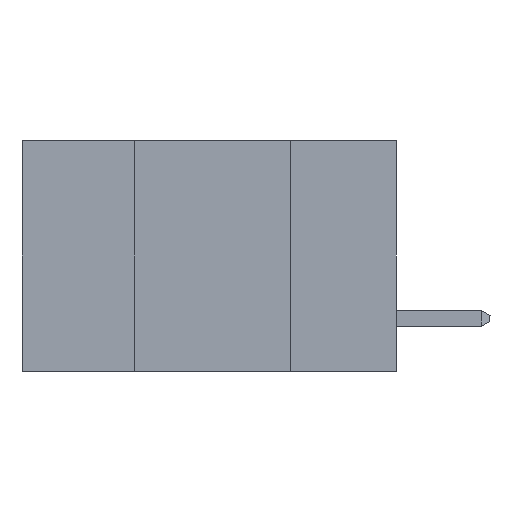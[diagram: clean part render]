
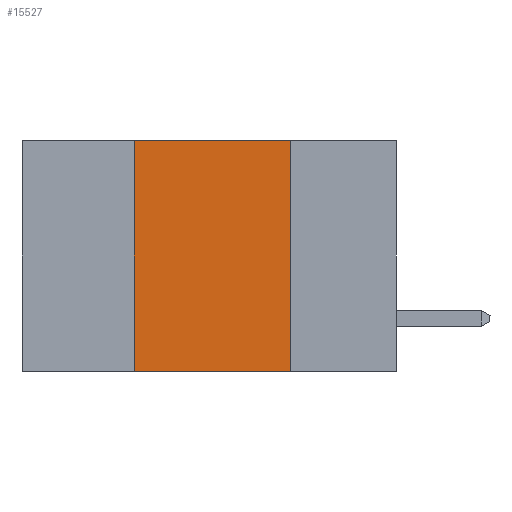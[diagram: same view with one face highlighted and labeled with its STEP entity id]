
A CAD part, left-side view. The second image highlights one B-rep face of the part: STEP entity #15527.
In plain terms, the highlighted planar face has unit normal (-1, 0, 0).
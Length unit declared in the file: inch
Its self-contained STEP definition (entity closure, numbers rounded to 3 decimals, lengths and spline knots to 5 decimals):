
#452 = VERTEX_POINT ( 'NONE', #5935 ) ;
#895 = DIRECTION ( 'NONE',  ( 0., 0., -1. ) ) ;
#1209 = DIRECTION ( 'NONE',  ( 0., 0., 1. ) ) ;
#1271 = CARTESIAN_POINT ( 'NONE',  ( 0., 0.42, -0.37 ) ) ;
#1286 = CARTESIAN_POINT ( 'NONE',  ( 0., 0.17, -0.37 ) ) ;
#2595 = AXIS2_PLACEMENT_3D ( 'NONE', #13153, #9141, #895 ) ;
#3821 = LINE ( 'NONE', #1271, #7104 ) ;
#4540 = ORIENTED_EDGE ( 'NONE', *, *, #9787, .F. ) ;
#4934 = FACE_OUTER_BOUND ( 'NONE', #7596, .T. ) ;
#5168 = VERTEX_POINT ( 'NONE', #16730 ) ;
#5935 = CARTESIAN_POINT ( 'NONE',  ( 0., 0.17, 0. ) ) ;
#6124 = VERTEX_POINT ( 'NONE', #9010 ) ;
#6601 = CARTESIAN_POINT ( 'NONE',  ( 0., 0.6, 0. ) ) ;
#6754 = CARTESIAN_POINT ( 'NONE',  ( 0., 0.6, -0.37 ) ) ;
#7034 = EDGE_CURVE ( 'NONE', #6124, #16229, #3821, .T. ) ;
#7104 = VECTOR ( 'NONE', #1209, 39.37008 ) ;
#7485 = LINE ( 'NONE', #6754, #11092 ) ;
#7596 = EDGE_LOOP ( 'NONE', ( #4540, #10369, #15245, #8282 ) ) ;
#7647 = LINE ( 'NONE', #1286, #13158 ) ;
#7778 = PLANE ( 'NONE',  #2595 ) ;
#8282 = ORIENTED_EDGE ( 'NONE', *, *, #11571, .T. ) ;
#9010 = CARTESIAN_POINT ( 'NONE',  ( 0., 0.42, -0.37 ) ) ;
#9141 = DIRECTION ( 'NONE',  ( 1., 0., 0. ) ) ;
#9295 = CARTESIAN_POINT ( 'NONE',  ( 0., 0.42, 0. ) ) ;
#9787 = EDGE_CURVE ( 'NONE', #452, #5168, #7647, .T. ) ;
#10369 = ORIENTED_EDGE ( 'NONE', *, *, #14325, .F. ) ;
#11092 = VECTOR ( 'NONE', #14893, 39.37008 ) ;
#11415 = LINE ( 'NONE', #6601, #11858 ) ;
#11571 = EDGE_CURVE ( 'NONE', #6124, #5168, #7485, .T. ) ;
#11858 = VECTOR ( 'NONE', #17416, 39.37008 ) ;
#13153 = CARTESIAN_POINT ( 'NONE',  ( 0., 0.6, 0. ) ) ;
#13158 = VECTOR ( 'NONE', #17615, 39.37008 ) ;
#14325 = EDGE_CURVE ( 'NONE', #16229, #452, #11415, .T. ) ;
#14893 = DIRECTION ( 'NONE',  ( 0., -1., 0. ) ) ;
#15245 = ORIENTED_EDGE ( 'NONE', *, *, #7034, .F. ) ;
#15527 = ADVANCED_FACE ( 'NONE', ( #4934 ), #7778, .F. ) ;
#16229 = VERTEX_POINT ( 'NONE', #9295 ) ;
#16730 = CARTESIAN_POINT ( 'NONE',  ( 0., 0.17, -0.37 ) ) ;
#17416 = DIRECTION ( 'NONE',  ( 0., -1., 0. ) ) ;
#17615 = DIRECTION ( 'NONE',  ( 0., 0., -1. ) ) ;
